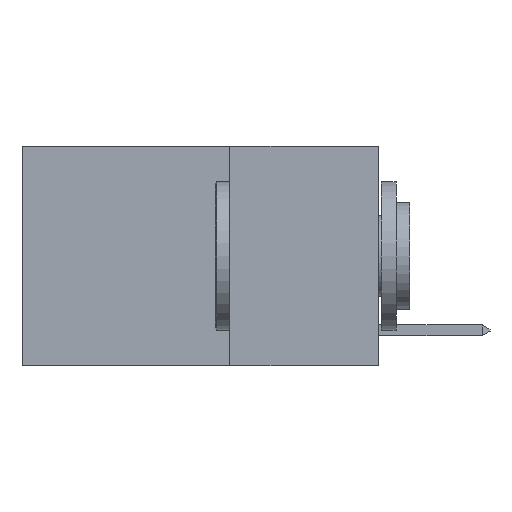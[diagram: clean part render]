
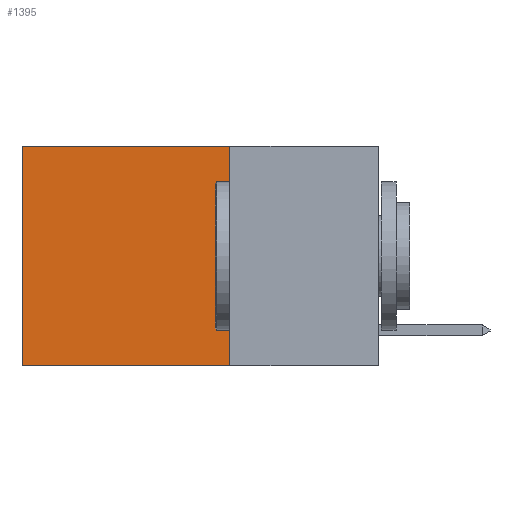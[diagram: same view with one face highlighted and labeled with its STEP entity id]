
A CAD part, left-side view. The second image highlights one B-rep face of the part: STEP entity #1395.
In plain terms, the highlighted planar face has unit normal (-1, 0, 0).
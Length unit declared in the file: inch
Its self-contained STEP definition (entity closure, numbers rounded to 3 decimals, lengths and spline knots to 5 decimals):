
#26 = VERTEX_POINT ( 'NONE', #9128 ) ;
#706 = EDGE_CURVE ( 'NONE', #8585, #26, #1538, .T. ) ;
#1103 = EDGE_CURVE ( 'NONE', #2307, #26, #2930, .T. ) ;
#1395 = ADVANCED_FACE ( 'NONE', ( #4049 ), #7154, .F. ) ;
#1538 = LINE ( 'NONE', #8801, #5999 ) ;
#2307 = VERTEX_POINT ( 'NONE', #2517 ) ;
#2442 = LINE ( 'NONE', #5478, #10739 ) ;
#2517 = CARTESIAN_POINT ( 'NONE',  ( 0.2625, 0.25, -0.37 ) ) ;
#2930 = LINE ( 'NONE', #8848, #7118 ) ;
#3779 = CARTESIAN_POINT ( 'NONE',  ( 0.2625, 0.25, 0. ) ) ;
#4049 = FACE_OUTER_BOUND ( 'NONE', #5930, .T. ) ;
#4432 = CARTESIAN_POINT ( 'NONE',  ( 0.2625, 0.6, 0. ) ) ;
#4615 = DIRECTION ( 'NONE',  ( 0., 1., 0. ) ) ;
#4676 = ORIENTED_EDGE ( 'NONE', *, *, #8810, .F. ) ;
#4778 = VECTOR ( 'NONE', #4615, 39.37008 ) ;
#5478 = CARTESIAN_POINT ( 'NONE',  ( 0.2625, 0.25, 0. ) ) ;
#5855 = EDGE_CURVE ( 'NONE', #10117, #8585, #7202, .T. ) ;
#5930 = EDGE_LOOP ( 'NONE', ( #8620, #10629, #4676, #6848 ) ) ;
#5999 = VECTOR ( 'NONE', #9122, 39.37008 ) ;
#6351 = DIRECTION ( 'NONE',  ( 0., 0., -1. ) ) ;
#6381 = DIRECTION ( 'NONE',  ( 1., 0., 0. ) ) ;
#6848 = ORIENTED_EDGE ( 'NONE', *, *, #5855, .T. ) ;
#6902 = CARTESIAN_POINT ( 'NONE',  ( 0.2625, 0.25, 0. ) ) ;
#7118 = VECTOR ( 'NONE', #10085, 39.37008 ) ;
#7154 = PLANE ( 'NONE',  #10602 ) ;
#7202 = LINE ( 'NONE', #3779, #4778 ) ;
#8585 = VERTEX_POINT ( 'NONE', #4432 ) ;
#8620 = ORIENTED_EDGE ( 'NONE', *, *, #706, .T. ) ;
#8797 = CARTESIAN_POINT ( 'NONE',  ( 0.2625, 0.25, 0. ) ) ;
#8801 = CARTESIAN_POINT ( 'NONE',  ( 0.2625, 0.6, 0. ) ) ;
#8810 = EDGE_CURVE ( 'NONE', #10117, #2307, #2442, .T. ) ;
#8848 = CARTESIAN_POINT ( 'NONE',  ( 0.2625, 0.25, -0.37 ) ) ;
#9122 = DIRECTION ( 'NONE',  ( 0., 0., -1. ) ) ;
#9128 = CARTESIAN_POINT ( 'NONE',  ( 0.2625, 0.6, -0.37 ) ) ;
#9327 = DIRECTION ( 'NONE',  ( 0., 0., -1. ) ) ;
#10085 = DIRECTION ( 'NONE',  ( 0., 1., 0. ) ) ;
#10117 = VERTEX_POINT ( 'NONE', #8797 ) ;
#10602 = AXIS2_PLACEMENT_3D ( 'NONE', #6902, #6381, #6351 ) ;
#10629 = ORIENTED_EDGE ( 'NONE', *, *, #1103, .F. ) ;
#10739 = VECTOR ( 'NONE', #9327, 39.37008 ) ;
